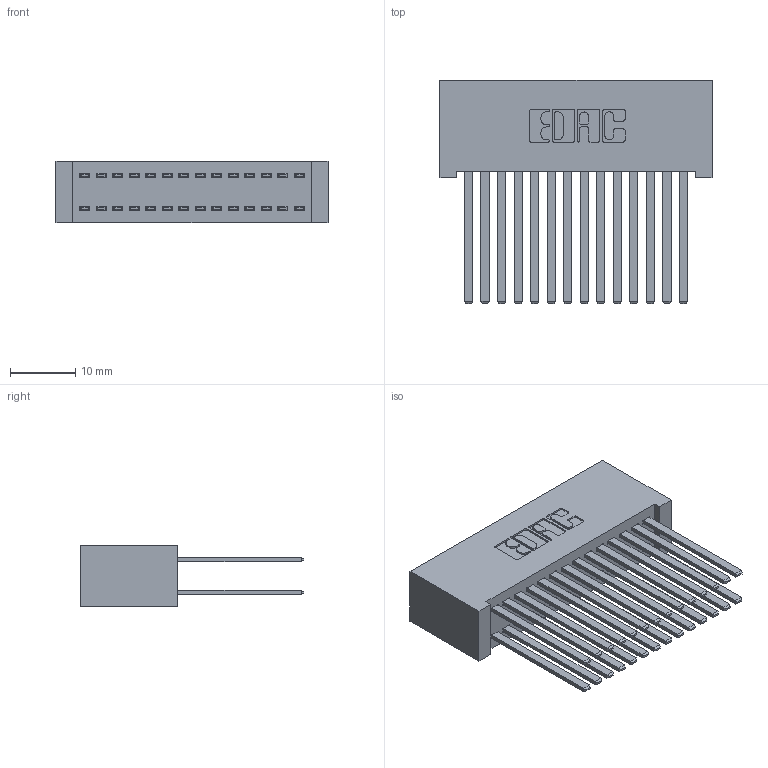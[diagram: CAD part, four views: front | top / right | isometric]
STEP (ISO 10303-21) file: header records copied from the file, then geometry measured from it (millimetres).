
FILE_DESCRIPTION (( 'STEP AP203' ), '1' );
FILE_NAME ('342-028-544-201.STEP', '2018-08-11T14:22:22', ( '' ), ( '' ), 'SwSTEP 2.0', 'SolidWorks 2016', '' );
FILE_SCHEMA (( 'CONFIG_CONTROL_DESIGN' ));
Length unit declared in the file: inch
Products named in the file (3): 342 Part_Lugless; 345-292-001_345-293-144; 342-028-544-201
Assembly tree (29 placements, depth 2):
  342-028-544-201
    342 Part_Lugless
    345-292-001_345-293-144  x28
Bounding box: 41.81 x 34.3 x 9.4 mm (x, y, z)
Volume: 4456 mm3; surface area: 8096.5 mm2
Topology: 29 solids, 29 shells, 1390 faces, 4111 edges, 2702 vertices
Faces by surface type: plane 958, cylinder 432
Entity records: 12035 total; most frequent: CARTESIAN_POINT 2022, ORIENTED_EDGE 1958, DIRECTION 1767, EDGE_CURVE 979, VECTOR 863, LINE 863, VERTEX_POINT 650, AXIS2_PLACEMENT_3D 452
